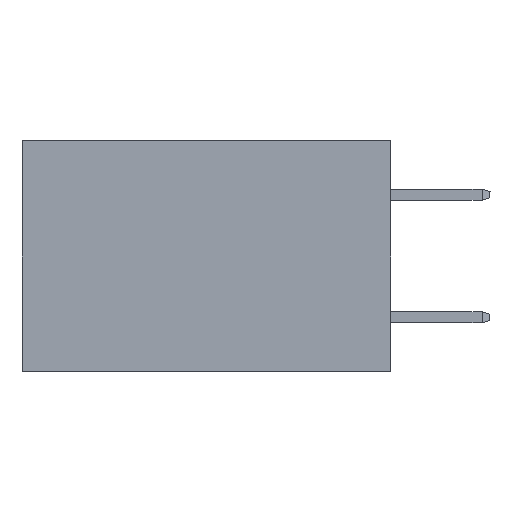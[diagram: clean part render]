
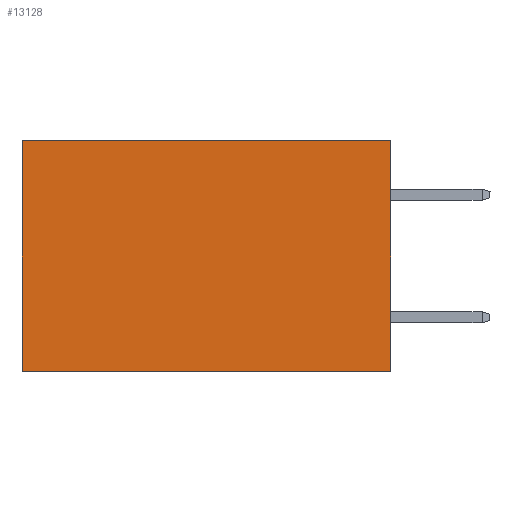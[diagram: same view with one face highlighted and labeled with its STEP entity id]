
A CAD part, left-side view. The second image highlights one B-rep face of the part: STEP entity #13128.
In plain terms, the highlighted planar face has unit normal (-1, 0, 0).
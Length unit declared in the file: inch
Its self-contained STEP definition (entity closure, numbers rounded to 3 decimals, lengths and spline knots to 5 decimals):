
#129 = PLANE ( 'NONE',  #6415 ) ;
#457 = CARTESIAN_POINT ( 'NONE',  ( 0.2875, 0., -0.375 ) ) ;
#940 = LINE ( 'NONE', #4008, #8405 ) ;
#953 = CARTESIAN_POINT ( 'NONE',  ( 0.2875, 0.6, -0.375 ) ) ;
#1546 = EDGE_CURVE ( 'NONE', #1628, #2058, #940, .T. ) ;
#1613 = CARTESIAN_POINT ( 'NONE',  ( 0.2875, 0., 0. ) ) ;
#1628 = VERTEX_POINT ( 'NONE', #3187 ) ;
#2058 = VERTEX_POINT ( 'NONE', #953 ) ;
#2233 = DIRECTION ( 'NONE',  ( 0., 0., -1. ) ) ;
#2610 = EDGE_CURVE ( 'NONE', #2623, #2058, #3461, .T. ) ;
#2623 = VERTEX_POINT ( 'NONE', #10615 ) ;
#2740 = VECTOR ( 'NONE', #6452, 39.37008 ) ;
#3020 = DIRECTION ( 'NONE',  ( 0., 0., -1. ) ) ;
#3187 = CARTESIAN_POINT ( 'NONE',  ( 0.2875, 0.6, 0. ) ) ;
#3461 = LINE ( 'NONE', #457, #2740 ) ;
#4008 = CARTESIAN_POINT ( 'NONE',  ( 0.2875, 0.6, -0.375 ) ) ;
#5664 = ORIENTED_EDGE ( 'NONE', *, *, #6076, .F. ) ;
#6076 = EDGE_CURVE ( 'NONE', #7219, #2623, #7104, .T. ) ;
#6415 = AXIS2_PLACEMENT_3D ( 'NONE', #7408, #7471, #2233 ) ;
#6452 = DIRECTION ( 'NONE',  ( 0., 1., 0. ) ) ;
#6810 = DIRECTION ( 'NONE',  ( 0., 1., 0. ) ) ;
#7095 = ORIENTED_EDGE ( 'NONE', *, *, #2610, .F. ) ;
#7104 = LINE ( 'NONE', #7235, #8006 ) ;
#7219 = VERTEX_POINT ( 'NONE', #1613 ) ;
#7235 = CARTESIAN_POINT ( 'NONE',  ( 0.2875, 0., -0.375 ) ) ;
#7339 = VECTOR ( 'NONE', #6810, 39.37008 ) ;
#7408 = CARTESIAN_POINT ( 'NONE',  ( 0.2875, 0., -0.375 ) ) ;
#7471 = DIRECTION ( 'NONE',  ( 1., 0., 0. ) ) ;
#8006 = VECTOR ( 'NONE', #3020, 39.37008 ) ;
#8109 = EDGE_CURVE ( 'NONE', #7219, #1628, #11937, .T. ) ;
#8156 = DIRECTION ( 'NONE',  ( 0., 0., -1. ) ) ;
#8405 = VECTOR ( 'NONE', #8156, 39.37008 ) ;
#8503 = FACE_OUTER_BOUND ( 'NONE', #9884, .T. ) ;
#9884 = EDGE_LOOP ( 'NONE', ( #10536, #7095, #5664, #13179 ) ) ;
#10536 = ORIENTED_EDGE ( 'NONE', *, *, #1546, .T. ) ;
#10615 = CARTESIAN_POINT ( 'NONE',  ( 0.2875, 0., -0.375 ) ) ;
#10849 = CARTESIAN_POINT ( 'NONE',  ( 0.2875, 0., 0. ) ) ;
#11937 = LINE ( 'NONE', #10849, #7339 ) ;
#13128 = ADVANCED_FACE ( 'NONE', ( #8503 ), #129, .F. ) ;
#13179 = ORIENTED_EDGE ( 'NONE', *, *, #8109, .T. ) ;
